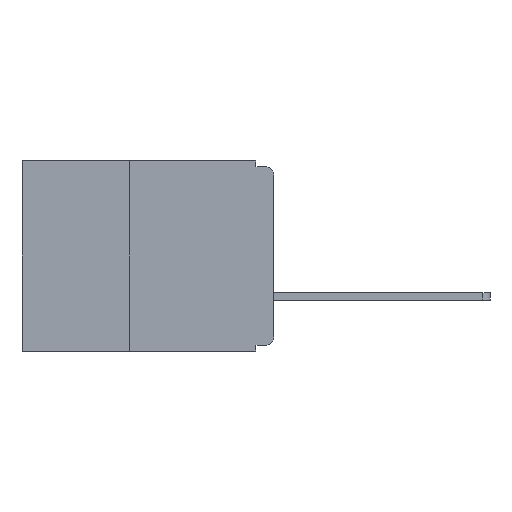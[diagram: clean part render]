
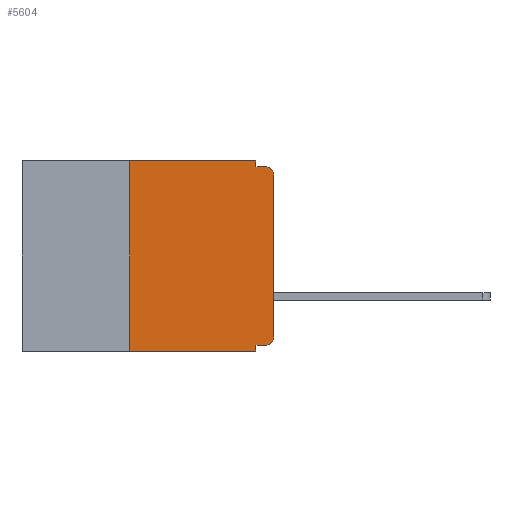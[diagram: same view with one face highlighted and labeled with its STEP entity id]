
A CAD part, left-side view. The second image highlights one B-rep face of the part: STEP entity #5604.
In plain terms, the highlighted planar face has unit normal (-1, 0, 0).
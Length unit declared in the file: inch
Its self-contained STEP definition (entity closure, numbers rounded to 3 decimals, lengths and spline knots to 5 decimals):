
#515 = LINE ( 'NONE', #4463, #20381 ) ;
#903 = CARTESIAN_POINT ( 'NONE',  ( 0., 0.031, -0.32 ) ) ;
#1309 = DIRECTION ( 'NONE',  ( -1., 0., 0. ) ) ;
#1495 = CARTESIAN_POINT ( 'NONE',  ( 0., 0.015, -0.32 ) ) ;
#1946 = ORIENTED_EDGE ( 'NONE', *, *, #15206, .T. ) ;
#2128 = ORIENTED_EDGE ( 'NONE', *, *, #26296, .F. ) ;
#3371 = ORIENTED_EDGE ( 'NONE', *, *, #19052, .F. ) ;
#3539 = ORIENTED_EDGE ( 'NONE', *, *, #17454, .T. ) ;
#4463 = CARTESIAN_POINT ( 'NONE',  ( 0., 0.437, -0.33 ) ) ;
#4505 = EDGE_CURVE ( 'NONE', #23201, #16066, #29255, .T. ) ;
#5439 = VERTEX_POINT ( 'NONE', #27934 ) ;
#5604 = ADVANCED_FACE ( 'NONE', ( #17169 ), #24769, .F. ) ;
#5626 = LINE ( 'NONE', #11579, #11774 ) ;
#5877 = CARTESIAN_POINT ( 'NONE',  ( 0., 0.031, -0.33 ) ) ;
#6243 = CARTESIAN_POINT ( 'NONE',  ( 0., 0.031, -0.01 ) ) ;
#6404 = DIRECTION ( 'NONE',  ( 0., 0., -1. ) ) ;
#6752 = ORIENTED_EDGE ( 'NONE', *, *, #29297, .F. ) ;
#7141 = EDGE_CURVE ( 'NONE', #9455, #14173, #28272, .T. ) ;
#8766 = CARTESIAN_POINT ( 'NONE',  ( 0., 0., -0.01 ) ) ;
#9455 = VERTEX_POINT ( 'NONE', #15684 ) ;
#9506 = DIRECTION ( 'NONE',  ( -1., 0., 0. ) ) ;
#9563 = CARTESIAN_POINT ( 'NONE',  ( 0., 0., 0. ) ) ;
#9794 = DIRECTION ( 'NONE',  ( 0., 0., 1. ) ) ;
#9884 = DIRECTION ( 'NONE',  ( 0., 0., 1. ) ) ;
#11253 = ORIENTED_EDGE ( 'NONE', *, *, #26303, .T. ) ;
#11321 = LINE ( 'NONE', #19356, #19671 ) ;
#11486 = ORIENTED_EDGE ( 'NONE', *, *, #4505, .F. ) ;
#11522 = VECTOR ( 'NONE', #9884, 39.37008 ) ;
#11579 = CARTESIAN_POINT ( 'NONE',  ( 0., 0.031, -0.33 ) ) ;
#11669 = VERTEX_POINT ( 'NONE', #5877 ) ;
#11774 = VECTOR ( 'NONE', #6404, 39.37008 ) ;
#12130 = CIRCLE ( 'NONE', #18010, 0.015 ) ;
#12410 = DIRECTION ( 'NONE',  ( 0., -1., 0. ) ) ;
#13323 = VECTOR ( 'NONE', #31850, 39.37008 ) ;
#13876 = CIRCLE ( 'NONE', #19660, 0.015 ) ;
#14173 = VERTEX_POINT ( 'NONE', #27685 ) ;
#14395 = CARTESIAN_POINT ( 'NONE',  ( 0., 0.25, 0. ) ) ;
#14908 = CARTESIAN_POINT ( 'NONE',  ( 0., 0.25, -0.33 ) ) ;
#15051 = VECTOR ( 'NONE', #9794, 39.37008 ) ;
#15175 = VECTOR ( 'NONE', #23899, 39.37008 ) ;
#15206 = EDGE_CURVE ( 'NONE', #16184, #9455, #13876, .T. ) ;
#15217 = LINE ( 'NONE', #22394, #27667 ) ;
#15684 = CARTESIAN_POINT ( 'NONE',  ( 0., 0., -0.305 ) ) ;
#16066 = VERTEX_POINT ( 'NONE', #6243 ) ;
#16184 = VERTEX_POINT ( 'NONE', #1495 ) ;
#16608 = CARTESIAN_POINT ( 'NONE',  ( 0., 0.015, -0.01 ) ) ;
#16703 = VERTEX_POINT ( 'NONE', #16608 ) ;
#16784 = VERTEX_POINT ( 'NONE', #14395 ) ;
#16900 = CARTESIAN_POINT ( 'NONE',  ( 0., 0.015, -0.305 ) ) ;
#17169 = FACE_OUTER_BOUND ( 'NONE', #20087, .T. ) ;
#17454 = EDGE_CURVE ( 'NONE', #14173, #16703, #12130, .T. ) ;
#17942 = EDGE_CURVE ( 'NONE', #16066, #16703, #32621, .T. ) ;
#18010 = AXIS2_PLACEMENT_3D ( 'NONE', #24569, #9506, #27061 ) ;
#19052 = EDGE_CURVE ( 'NONE', #5439, #16784, #24829, .T. ) ;
#19356 = CARTESIAN_POINT ( 'NONE',  ( 0., 0., -0.32 ) ) ;
#19453 = DIRECTION ( 'NONE',  ( 0., 0., -1. ) ) ;
#19660 = AXIS2_PLACEMENT_3D ( 'NONE', #16900, #1309, #19453 ) ;
#19671 = VECTOR ( 'NONE', #21853, 39.37008 ) ;
#20087 = EDGE_LOOP ( 'NONE', ( #30778, #3539, #23936, #11486, #2128, #3371, #11253, #6752, #31003, #1946 ) ) ;
#20381 = VECTOR ( 'NONE', #29799, 39.37008 ) ;
#21853 = DIRECTION ( 'NONE',  ( 0., 1., 0. ) ) ;
#22394 = CARTESIAN_POINT ( 'NONE',  ( 0., 0.437, 0. ) ) ;
#23201 = VERTEX_POINT ( 'NONE', #27806 ) ;
#23508 = VERTEX_POINT ( 'NONE', #903 ) ;
#23899 = DIRECTION ( 'NONE',  ( 0., -1., 0. ) ) ;
#23936 = ORIENTED_EDGE ( 'NONE', *, *, #17942, .F. ) ;
#24569 = CARTESIAN_POINT ( 'NONE',  ( 0., 0.015, -0.025 ) ) ;
#24655 = DIRECTION ( 'NONE',  ( 0., 0., -1. ) ) ;
#24684 = DIRECTION ( 'NONE',  ( 1., 0., 0. ) ) ;
#24769 = PLANE ( 'NONE',  #26101 ) ;
#24829 = LINE ( 'NONE', #14908, #11522 ) ;
#24982 = CARTESIAN_POINT ( 'NONE',  ( 0., 0.437, 0. ) ) ;
#26101 = AXIS2_PLACEMENT_3D ( 'NONE', #24982, #24684, #24655 ) ;
#26296 = EDGE_CURVE ( 'NONE', #16784, #23201, #15217, .T. ) ;
#26303 = EDGE_CURVE ( 'NONE', #5439, #11669, #515, .T. ) ;
#27061 = DIRECTION ( 'NONE',  ( 0., 0., -1. ) ) ;
#27667 = VECTOR ( 'NONE', #12410, 39.37008 ) ;
#27685 = CARTESIAN_POINT ( 'NONE',  ( 0., 0., -0.025 ) ) ;
#27806 = CARTESIAN_POINT ( 'NONE',  ( 0., 0.031, 0. ) ) ;
#27934 = CARTESIAN_POINT ( 'NONE',  ( 0., 0.25, -0.33 ) ) ;
#28272 = LINE ( 'NONE', #9563, #15051 ) ;
#29255 = LINE ( 'NONE', #31892, #13323 ) ;
#29297 = EDGE_CURVE ( 'NONE', #23508, #11669, #5626, .T. ) ;
#29799 = DIRECTION ( 'NONE',  ( 0., -1., 0. ) ) ;
#29974 = EDGE_CURVE ( 'NONE', #16184, #23508, #11321, .T. ) ;
#30778 = ORIENTED_EDGE ( 'NONE', *, *, #7141, .T. ) ;
#31003 = ORIENTED_EDGE ( 'NONE', *, *, #29974, .F. ) ;
#31850 = DIRECTION ( 'NONE',  ( 0., 0., -1. ) ) ;
#31892 = CARTESIAN_POINT ( 'NONE',  ( 0., 0.031, 0. ) ) ;
#32621 = LINE ( 'NONE', #8766, #15175 ) ;
